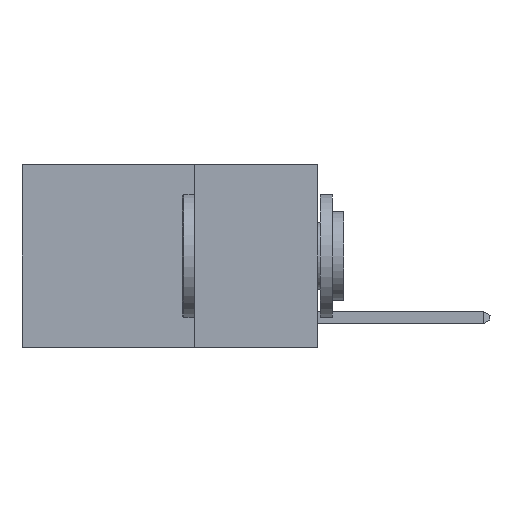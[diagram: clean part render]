
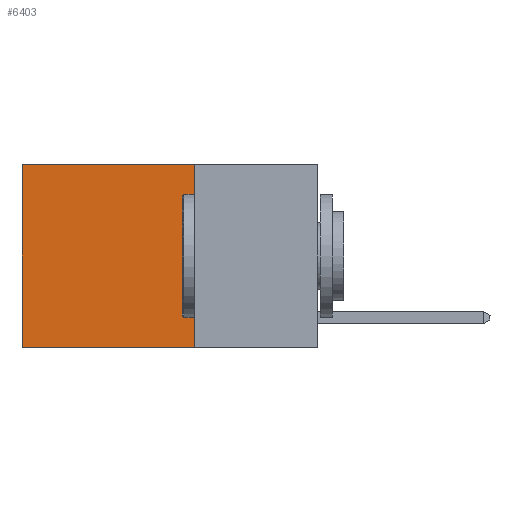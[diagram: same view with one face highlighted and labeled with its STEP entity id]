
A CAD part, left-side view. The second image highlights one B-rep face of the part: STEP entity #6403.
In plain terms, the highlighted planar face has unit normal (-1, 0, 0).
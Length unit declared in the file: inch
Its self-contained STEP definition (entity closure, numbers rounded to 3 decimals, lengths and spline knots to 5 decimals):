
#124 = EDGE_CURVE ( 'NONE', #11004, #8979, #15780, .T. ) ;
#1334 = EDGE_CURVE ( 'NONE', #4683, #11004, #6846, .T. ) ;
#2192 = VECTOR ( 'NONE', #3241, 39.37008 ) ;
#2541 = DIRECTION ( 'NONE',  ( 0., 0., -1. ) ) ;
#2622 = LINE ( 'NONE', #10560, #16188 ) ;
#2631 = DIRECTION ( 'NONE',  ( 0., 0., -1. ) ) ;
#2770 = CARTESIAN_POINT ( 'NONE',  ( 0.2625, 0.25, 0. ) ) ;
#3241 = DIRECTION ( 'NONE',  ( 0., 1., 0. ) ) ;
#3763 = ORIENTED_EDGE ( 'NONE', *, *, #1334, .F. ) ;
#3772 = PLANE ( 'NONE',  #5170 ) ;
#4225 = VERTEX_POINT ( 'NONE', #11444 ) ;
#4683 = VERTEX_POINT ( 'NONE', #12461 ) ;
#4710 = DIRECTION ( 'NONE',  ( 0., 1., 0. ) ) ;
#4855 = ORIENTED_EDGE ( 'NONE', *, *, #10911, .T. ) ;
#5130 = DIRECTION ( 'NONE',  ( 0., 0., -1. ) ) ;
#5170 = AXIS2_PLACEMENT_3D ( 'NONE', #15548, #12991, #5130 ) ;
#6218 = CARTESIAN_POINT ( 'NONE',  ( 0.2625, 0.25, -0.37 ) ) ;
#6403 = ADVANCED_FACE ( 'NONE', ( #10181 ), #3772, .F. ) ;
#6846 = LINE ( 'NONE', #2770, #13844 ) ;
#8029 = ORIENTED_EDGE ( 'NONE', *, *, #11819, .T. ) ;
#8979 = VERTEX_POINT ( 'NONE', #11652 ) ;
#10181 = FACE_OUTER_BOUND ( 'NONE', #13837, .T. ) ;
#10283 = ORIENTED_EDGE ( 'NONE', *, *, #124, .F. ) ;
#10560 = CARTESIAN_POINT ( 'NONE',  ( 0.2625, 0.6, 0. ) ) ;
#10911 = EDGE_CURVE ( 'NONE', #4683, #4225, #16217, .T. ) ;
#11004 = VERTEX_POINT ( 'NONE', #6218 ) ;
#11205 = CARTESIAN_POINT ( 'NONE',  ( 0.2625, 0.25, -0.37 ) ) ;
#11444 = CARTESIAN_POINT ( 'NONE',  ( 0.2625, 0.6, 0. ) ) ;
#11652 = CARTESIAN_POINT ( 'NONE',  ( 0.2625, 0.6, -0.37 ) ) ;
#11819 = EDGE_CURVE ( 'NONE', #4225, #8979, #2622, .T. ) ;
#12461 = CARTESIAN_POINT ( 'NONE',  ( 0.2625, 0.25, 0. ) ) ;
#12762 = VECTOR ( 'NONE', #4710, 39.37008 ) ;
#12991 = DIRECTION ( 'NONE',  ( 1., 0., 0. ) ) ;
#13837 = EDGE_LOOP ( 'NONE', ( #8029, #10283, #3763, #4855 ) ) ;
#13844 = VECTOR ( 'NONE', #2541, 39.37008 ) ;
#13924 = CARTESIAN_POINT ( 'NONE',  ( 0.2625, 0.25, 0. ) ) ;
#15548 = CARTESIAN_POINT ( 'NONE',  ( 0.2625, 0.25, 0. ) ) ;
#15780 = LINE ( 'NONE', #11205, #2192 ) ;
#16188 = VECTOR ( 'NONE', #2631, 39.37008 ) ;
#16217 = LINE ( 'NONE', #13924, #12762 ) ;
